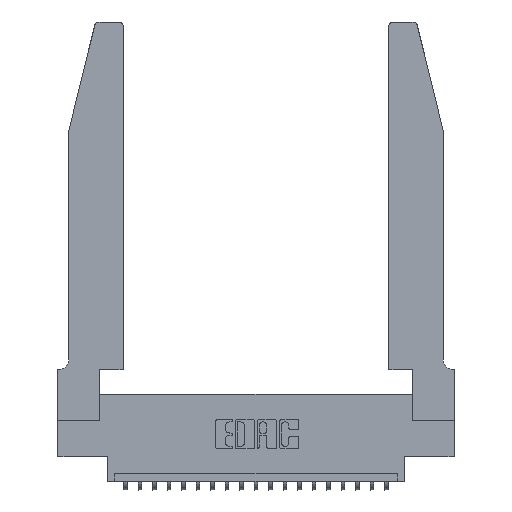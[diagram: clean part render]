
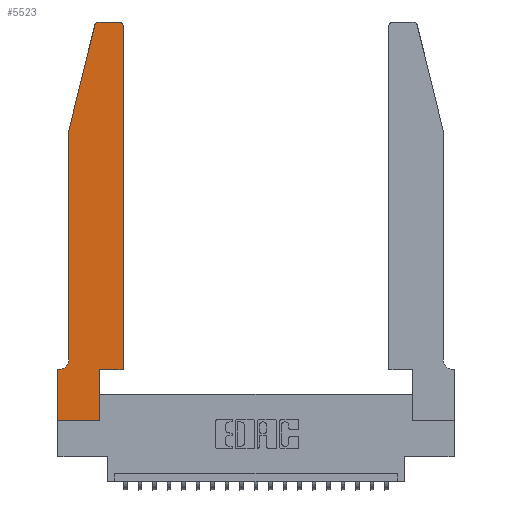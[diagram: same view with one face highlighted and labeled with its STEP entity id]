
A CAD part, top view. The second image highlights one B-rep face of the part: STEP entity #5523.
In plain terms, the highlighted planar face has unit normal (0, 0, 1).
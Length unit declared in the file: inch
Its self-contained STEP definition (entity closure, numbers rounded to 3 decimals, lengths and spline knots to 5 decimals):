
#178 = LINE ( 'NONE', #6465, #21781 ) ;
#300 = CARTESIAN_POINT ( 'NONE',  ( 0.0755, 2., 0.37 ) ) ;
#314 = CARTESIAN_POINT ( 'NONE',  ( 0.25487, 2.72718, 0.37 ) ) ;
#607 = CARTESIAN_POINT ( 'NONE',  ( 0.4505, 0.35, 0.37 ) ) ;
#655 = ORIENTED_EDGE ( 'NONE', *, *, #16837, .T. ) ;
#752 = ORIENTED_EDGE ( 'NONE', *, *, #20691, .T. ) ;
#1162 = DIRECTION ( 'NONE',  ( 0., 0., 1. ) ) ;
#1432 = CARTESIAN_POINT ( 'NONE',  ( 0.0755, 2., 0.37 ) ) ;
#1486 = DIRECTION ( 'NONE',  ( 0., 0., 1. ) ) ;
#1870 = EDGE_CURVE ( 'NONE', #11279, #14177, #6654, .T. ) ;
#1942 = ORIENTED_EDGE ( 'NONE', *, *, #16873, .T. ) ;
#2071 = EDGE_CURVE ( 'NONE', #4828, #11279, #16647, .T. ) ;
#2394 = VERTEX_POINT ( 'NONE', #7873 ) ;
#2458 = CARTESIAN_POINT ( 'NONE',  ( 0., 0., 0.37 ) ) ;
#2466 = LINE ( 'NONE', #1432, #18930 ) ;
#2505 = ORIENTED_EDGE ( 'NONE', *, *, #11782, .T. ) ;
#2584 = VERTEX_POINT ( 'NONE', #10509 ) ;
#3836 = ORIENTED_EDGE ( 'NONE', *, *, #4366, .T. ) ;
#3952 = VECTOR ( 'NONE', #6221, 39.37008 ) ;
#4166 = DIRECTION ( 'NONE',  ( -1., 0., 0. ) ) ;
#4351 = CARTESIAN_POINT ( 'NONE',  ( 0., 0., 0.37 ) ) ;
#4366 = EDGE_CURVE ( 'NONE', #19806, #2394, #12479, .T. ) ;
#4368 = LINE ( 'NONE', #18142, #4635 ) ;
#4618 = VECTOR ( 'NONE', #7662, 39.37008 ) ;
#4635 = VECTOR ( 'NONE', #14799, 39.37008 ) ;
#4767 = VECTOR ( 'NONE', #14474, 39.37008 ) ;
#4828 = VERTEX_POINT ( 'NONE', #16997 ) ;
#4844 = ORIENTED_EDGE ( 'NONE', *, *, #16015, .T. ) ;
#5515 = VERTEX_POINT ( 'NONE', #16586 ) ;
#5523 = ADVANCED_FACE ( 'NONE', ( #5962 ), #22288, .T. ) ;
#5635 = ORIENTED_EDGE ( 'NONE', *, *, #17590, .T. ) ;
#5644 = ORIENTED_EDGE ( 'NONE', *, *, #21318, .T. ) ;
#5859 = VECTOR ( 'NONE', #13873, 39.37008 ) ;
#5962 = FACE_OUTER_BOUND ( 'NONE', #12513, .T. ) ;
#6058 = DIRECTION ( 'NONE',  ( 0., 0., -1. ) ) ;
#6156 = DIRECTION ( 'NONE',  ( 1., 0., 0. ) ) ;
#6221 = DIRECTION ( 'NONE',  ( -1., 0., 0. ) ) ;
#6241 = VERTEX_POINT ( 'NONE', #314 ) ;
#6465 = CARTESIAN_POINT ( 'NONE',  ( 0.0755, 2., 0.37 ) ) ;
#6540 = DIRECTION ( 'NONE',  ( 0., -1., 0. ) ) ;
#6654 = LINE ( 'NONE', #17242, #13148 ) ;
#6661 = LINE ( 'NONE', #11575, #18035 ) ;
#6698 = DIRECTION ( 'NONE',  ( -0.239, -0.971, 0. ) ) ;
#7432 = VERTEX_POINT ( 'NONE', #4351 ) ;
#7490 = CARTESIAN_POINT ( 'NONE',  ( 0.2605, 2.75, 0.37 ) ) ;
#7662 = DIRECTION ( 'NONE',  ( 0., -1., 0. ) ) ;
#7873 = CARTESIAN_POINT ( 'NONE',  ( 0.0055, 0.35, 0.37 ) ) ;
#8080 = AXIS2_PLACEMENT_3D ( 'NONE', #11511, #1162, #6156 ) ;
#8529 = LINE ( 'NONE', #7490, #3952 ) ;
#9379 = LINE ( 'NONE', #11032, #4767 ) ;
#10502 = ORIENTED_EDGE ( 'NONE', *, *, #14438, .T. ) ;
#10509 = CARTESIAN_POINT ( 'NONE',  ( 0.4205, 2.75, 0.37 ) ) ;
#11032 = CARTESIAN_POINT ( 'NONE',  ( 0.0755, 0.35, 0.37 ) ) ;
#11279 = VERTEX_POINT ( 'NONE', #16559 ) ;
#11369 = CARTESIAN_POINT ( 'NONE',  ( 0.284, 2.75, 0.37 ) ) ;
#11511 = CARTESIAN_POINT ( 'NONE',  ( 0.4205, 2.72, 0.37 ) ) ;
#11568 = ORIENTED_EDGE ( 'NONE', *, *, #13702, .T. ) ;
#11575 = CARTESIAN_POINT ( 'NONE',  ( 0.4505, 0.35, 0.37 ) ) ;
#11702 = DIRECTION ( 'NONE',  ( 0., 1., 0. ) ) ;
#11782 = EDGE_CURVE ( 'NONE', #2394, #14755, #9379, .T. ) ;
#12298 = DIRECTION ( 'NONE',  ( 0., 0., 1. ) ) ;
#12479 = CIRCLE ( 'NONE', #12861, 0.07 ) ;
#12513 = EDGE_LOOP ( 'NONE', ( #5635, #752, #11568, #655, #3836, #2505, #5644, #10502, #22018, #15639, #1942, #4844 ) ) ;
#12720 = AXIS2_PLACEMENT_3D ( 'NONE', #18699, #12298, #20792 ) ;
#12861 = AXIS2_PLACEMENT_3D ( 'NONE', #21504, #6058, #4166 ) ;
#13148 = VECTOR ( 'NONE', #15770, 39.37008 ) ;
#13702 = EDGE_CURVE ( 'NONE', #6241, #20005, #2466, .T. ) ;
#13873 = DIRECTION ( 'NONE',  ( 0., 1., 0. ) ) ;
#14177 = VERTEX_POINT ( 'NONE', #607 ) ;
#14369 = CIRCLE ( 'NONE', #19397, 0.03 ) ;
#14438 = EDGE_CURVE ( 'NONE', #7432, #4828, #4368, .T. ) ;
#14474 = DIRECTION ( 'NONE',  ( -1., 0., 0. ) ) ;
#14755 = VERTEX_POINT ( 'NONE', #17689 ) ;
#14799 = DIRECTION ( 'NONE',  ( 1., 0., 0. ) ) ;
#15591 = CARTESIAN_POINT ( 'NONE',  ( 0.0755, 0.42, 0.37 ) ) ;
#15639 = ORIENTED_EDGE ( 'NONE', *, *, #1870, .T. ) ;
#15770 = DIRECTION ( 'NONE',  ( 1., 0., 0. ) ) ;
#16015 = EDGE_CURVE ( 'NONE', #5515, #2584, #21268, .T. ) ;
#16036 = VERTEX_POINT ( 'NONE', #11369 ) ;
#16559 = CARTESIAN_POINT ( 'NONE',  ( 0.2865, 0.35, 0.37 ) ) ;
#16586 = CARTESIAN_POINT ( 'NONE',  ( 0.4505, 2.72, 0.37 ) ) ;
#16647 = LINE ( 'NONE', #19273, #5859 ) ;
#16770 = LINE ( 'NONE', #2458, #4618 ) ;
#16837 = EDGE_CURVE ( 'NONE', #20005, #19806, #178, .T. ) ;
#16873 = EDGE_CURVE ( 'NONE', #14177, #5515, #6661, .T. ) ;
#16997 = CARTESIAN_POINT ( 'NONE',  ( 0.2865, 0., 0.37 ) ) ;
#17242 = CARTESIAN_POINT ( 'NONE',  ( 0.4505, 0.35, 0.37 ) ) ;
#17590 = EDGE_CURVE ( 'NONE', #2584, #16036, #8529, .T. ) ;
#17689 = CARTESIAN_POINT ( 'NONE',  ( 0., 0.35, 0.37 ) ) ;
#18035 = VECTOR ( 'NONE', #11702, 39.37008 ) ;
#18142 = CARTESIAN_POINT ( 'NONE',  ( 0., 0., 0.37 ) ) ;
#18679 = DIRECTION ( 'NONE',  ( 1., 0., 0. ) ) ;
#18699 = CARTESIAN_POINT ( 'NONE',  ( 0., 0.35, 0.37 ) ) ;
#18930 = VECTOR ( 'NONE', #6698, 39.37008 ) ;
#19273 = CARTESIAN_POINT ( 'NONE',  ( 0.2865, 0.35, 0.37 ) ) ;
#19397 = AXIS2_PLACEMENT_3D ( 'NONE', #19735, #1486, #18679 ) ;
#19735 = CARTESIAN_POINT ( 'NONE',  ( 0.284, 2.72, 0.37 ) ) ;
#19806 = VERTEX_POINT ( 'NONE', #15591 ) ;
#20005 = VERTEX_POINT ( 'NONE', #300 ) ;
#20691 = EDGE_CURVE ( 'NONE', #16036, #6241, #14369, .T. ) ;
#20792 = DIRECTION ( 'NONE',  ( 1., 0., 0. ) ) ;
#21268 = CIRCLE ( 'NONE', #8080, 0.03 ) ;
#21318 = EDGE_CURVE ( 'NONE', #14755, #7432, #16770, .T. ) ;
#21504 = CARTESIAN_POINT ( 'NONE',  ( 0.0055, 0.42, 0.37 ) ) ;
#21781 = VECTOR ( 'NONE', #6540, 39.37008 ) ;
#22018 = ORIENTED_EDGE ( 'NONE', *, *, #2071, .T. ) ;
#22288 = PLANE ( 'NONE',  #12720 ) ;
